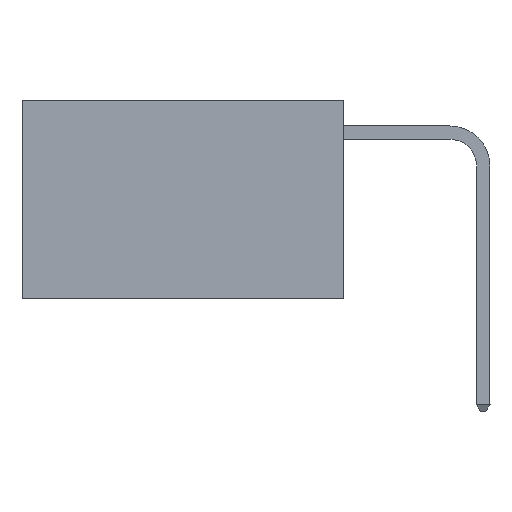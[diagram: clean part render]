
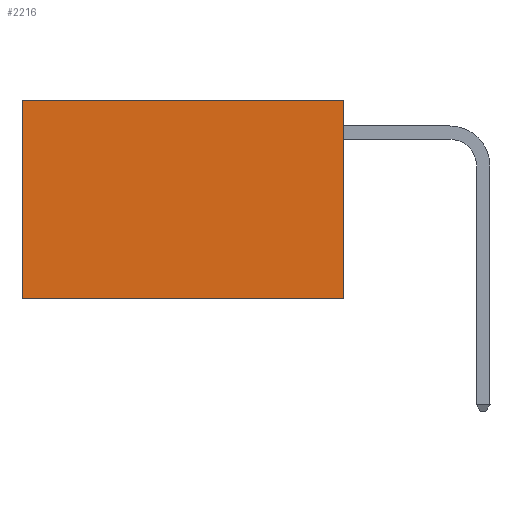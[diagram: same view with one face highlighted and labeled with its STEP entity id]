
A CAD part, left-side view. The second image highlights one B-rep face of the part: STEP entity #2216.
In plain terms, the highlighted planar face has unit normal (-1, 0, 0).
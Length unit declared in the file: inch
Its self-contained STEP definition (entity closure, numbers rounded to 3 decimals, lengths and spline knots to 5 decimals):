
#208 = VERTEX_POINT ( 'NONE', #14532 ) ;
#249 = DIRECTION ( 'NONE',  ( 0., 1., 0. ) ) ;
#2167 = CARTESIAN_POINT ( 'NONE',  ( 0.2625, 0.6, 0. ) ) ;
#2211 = FACE_OUTER_BOUND ( 'NONE', #9394, .T. ) ;
#2214 = VECTOR ( 'NONE', #5727, 39.37008 ) ;
#2216 = ADVANCED_FACE ( 'NONE', ( #2211 ), #14324, .F. ) ;
#2642 = EDGE_CURVE ( 'NONE', #8447, #208, #9122, .T. ) ;
#2955 = EDGE_CURVE ( 'NONE', #208, #11699, #14081, .T. ) ;
#4010 = CARTESIAN_POINT ( 'NONE',  ( 0.2625, 0., 0. ) ) ;
#4593 = VECTOR ( 'NONE', #249, 39.37008 ) ;
#4743 = CARTESIAN_POINT ( 'NONE',  ( 0.2625, 0., -0.37 ) ) ;
#5216 = DIRECTION ( 'NONE',  ( 0., 0., -1. ) ) ;
#5330 = LINE ( 'NONE', #14919, #4593 ) ;
#5372 = VECTOR ( 'NONE', #7862, 39.37008 ) ;
#5727 = DIRECTION ( 'NONE',  ( 0., 0., -1. ) ) ;
#5869 = EDGE_CURVE ( 'NONE', #6189, #11699, #5330, .T. ) ;
#6189 = VERTEX_POINT ( 'NONE', #4743 ) ;
#6444 = DIRECTION ( 'NONE',  ( 0., 1., 0. ) ) ;
#7862 = DIRECTION ( 'NONE',  ( 0., 0., -1. ) ) ;
#8011 = DIRECTION ( 'NONE',  ( 1., 0., 0. ) ) ;
#8447 = VERTEX_POINT ( 'NONE', #10595 ) ;
#9122 = LINE ( 'NONE', #4010, #12744 ) ;
#9128 = CARTESIAN_POINT ( 'NONE',  ( 0.2625, 0., 0. ) ) ;
#9244 = CARTESIAN_POINT ( 'NONE',  ( 0.2625, 0.6, -0.37 ) ) ;
#9394 = EDGE_LOOP ( 'NONE', ( #15047, #14903, #13038, #13176 ) ) ;
#10595 = CARTESIAN_POINT ( 'NONE',  ( 0.2625, 0., 0. ) ) ;
#11115 = AXIS2_PLACEMENT_3D ( 'NONE', #15421, #8011, #5216 ) ;
#11650 = EDGE_CURVE ( 'NONE', #8447, #6189, #15153, .T. ) ;
#11699 = VERTEX_POINT ( 'NONE', #9244 ) ;
#12744 = VECTOR ( 'NONE', #6444, 39.37008 ) ;
#13038 = ORIENTED_EDGE ( 'NONE', *, *, #11650, .F. ) ;
#13176 = ORIENTED_EDGE ( 'NONE', *, *, #2642, .T. ) ;
#14081 = LINE ( 'NONE', #2167, #2214 ) ;
#14324 = PLANE ( 'NONE',  #11115 ) ;
#14532 = CARTESIAN_POINT ( 'NONE',  ( 0.2625, 0.6, 0. ) ) ;
#14903 = ORIENTED_EDGE ( 'NONE', *, *, #5869, .F. ) ;
#14919 = CARTESIAN_POINT ( 'NONE',  ( 0.2625, 0., -0.37 ) ) ;
#15047 = ORIENTED_EDGE ( 'NONE', *, *, #2955, .T. ) ;
#15153 = LINE ( 'NONE', #9128, #5372 ) ;
#15421 = CARTESIAN_POINT ( 'NONE',  ( 0.2625, 0., 0. ) ) ;
